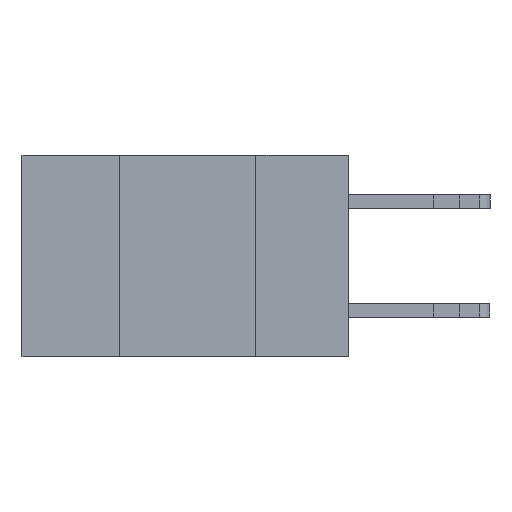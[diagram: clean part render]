
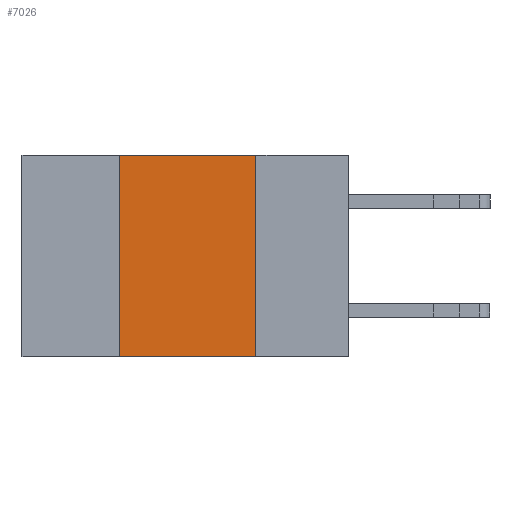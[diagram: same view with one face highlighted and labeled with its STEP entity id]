
A CAD part, left-side view. The second image highlights one B-rep face of the part: STEP entity #7026.
In plain terms, the highlighted planar face has unit normal (-1, 0, 0).
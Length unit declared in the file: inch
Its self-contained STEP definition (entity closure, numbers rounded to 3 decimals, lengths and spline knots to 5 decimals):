
#297 = ORIENTED_EDGE ( 'NONE', *, *, #5378, .T. ) ;
#661 = CARTESIAN_POINT ( 'NONE',  ( 0., 0.17, 0. ) ) ;
#920 = CARTESIAN_POINT ( 'NONE',  ( 0., 0.6, 0. ) ) ;
#1056 = CARTESIAN_POINT ( 'NONE',  ( 0., 0.17, 0. ) ) ;
#1793 = DIRECTION ( 'NONE',  ( 0., 0., -1. ) ) ;
#1934 = AXIS2_PLACEMENT_3D ( 'NONE', #920, #13564, #2731 ) ;
#2731 = DIRECTION ( 'NONE',  ( 0., 0., -1. ) ) ;
#2867 = VERTEX_POINT ( 'NONE', #3660 ) ;
#3660 = CARTESIAN_POINT ( 'NONE',  ( 0., 0.42, 0. ) ) ;
#5378 = EDGE_CURVE ( 'NONE', #11670, #14060, #12260, .T. ) ;
#5437 = VECTOR ( 'NONE', #1793, 39.37008 ) ;
#6477 = CARTESIAN_POINT ( 'NONE',  ( 0., 0.42, -0.37 ) ) ;
#7026 = ADVANCED_FACE ( 'NONE', ( #15805 ), #15254, .F. ) ;
#7283 = LINE ( 'NONE', #22685, #16268 ) ;
#7828 = EDGE_LOOP ( 'NONE', ( #10167, #8781, #11044, #297 ) ) ;
#8781 = ORIENTED_EDGE ( 'NONE', *, *, #10487, .F. ) ;
#9181 = CARTESIAN_POINT ( 'NONE',  ( 0., 0.42, 0. ) ) ;
#10167 = ORIENTED_EDGE ( 'NONE', *, *, #17292, .F. ) ;
#10487 = EDGE_CURVE ( 'NONE', #2867, #22623, #7283, .T. ) ;
#11044 = ORIENTED_EDGE ( 'NONE', *, *, #19849, .F. ) ;
#11670 = VERTEX_POINT ( 'NONE', #6477 ) ;
#12260 = LINE ( 'NONE', #19245, #17446 ) ;
#13564 = DIRECTION ( 'NONE',  ( 1., 0., 0. ) ) ;
#14060 = VERTEX_POINT ( 'NONE', #19654 ) ;
#14094 = DIRECTION ( 'NONE',  ( 0., -1., 0. ) ) ;
#15254 = PLANE ( 'NONE',  #1934 ) ;
#15805 = FACE_OUTER_BOUND ( 'NONE', #7828, .T. ) ;
#16268 = VECTOR ( 'NONE', #14094, 39.37008 ) ;
#16335 = DIRECTION ( 'NONE',  ( 0., 0., 1. ) ) ;
#16513 = VECTOR ( 'NONE', #16335, 39.37008 ) ;
#17292 = EDGE_CURVE ( 'NONE', #22623, #14060, #19621, .T. ) ;
#17446 = VECTOR ( 'NONE', #19552, 39.37008 ) ;
#19245 = CARTESIAN_POINT ( 'NONE',  ( 0., 0.6, -0.37 ) ) ;
#19552 = DIRECTION ( 'NONE',  ( 0., -1., 0. ) ) ;
#19621 = LINE ( 'NONE', #1056, #5437 ) ;
#19654 = CARTESIAN_POINT ( 'NONE',  ( 0., 0.17, -0.37 ) ) ;
#19849 = EDGE_CURVE ( 'NONE', #11670, #2867, #21108, .T. ) ;
#21108 = LINE ( 'NONE', #9181, #16513 ) ;
#22623 = VERTEX_POINT ( 'NONE', #661 ) ;
#22685 = CARTESIAN_POINT ( 'NONE',  ( 0., 0.6, 0. ) ) ;
